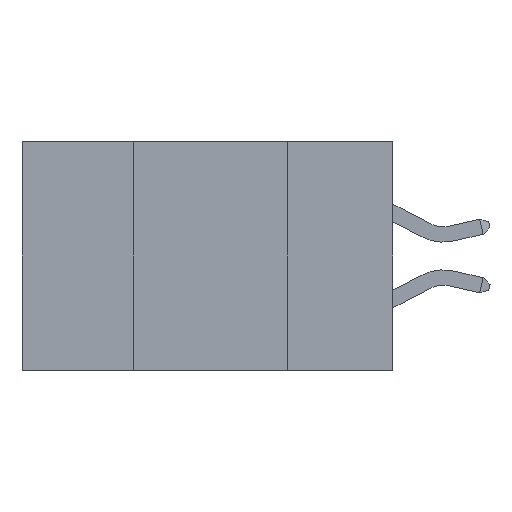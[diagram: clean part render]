
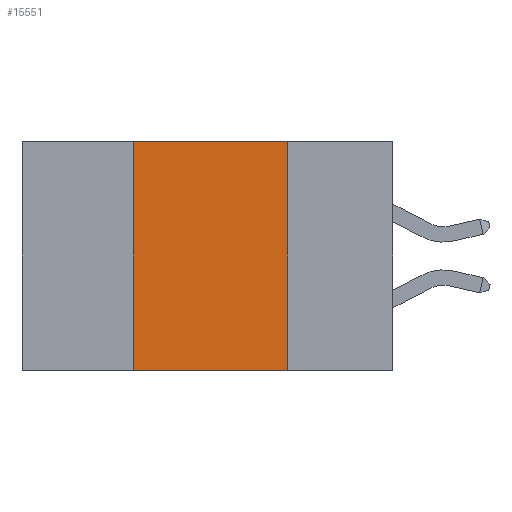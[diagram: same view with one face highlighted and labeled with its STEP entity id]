
A CAD part, left-side view. The second image highlights one B-rep face of the part: STEP entity #15551.
In plain terms, the highlighted planar face has unit normal (-1, 0, 0).
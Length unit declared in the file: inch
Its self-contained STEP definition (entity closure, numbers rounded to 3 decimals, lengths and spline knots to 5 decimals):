
#115 = CARTESIAN_POINT ( 'NONE',  ( 0., 0.17, 0. ) ) ;
#1339 = CARTESIAN_POINT ( 'NONE',  ( 0., 0.42, 0. ) ) ;
#2048 = LINE ( 'NONE', #1339, #14881 ) ;
#2567 = LINE ( 'NONE', #10502, #19224 ) ;
#3189 = EDGE_CURVE ( 'NONE', #14061, #12010, #2048, .T. ) ;
#3264 = VERTEX_POINT ( 'NONE', #9526 ) ;
#3727 = EDGE_LOOP ( 'NONE', ( #8977, #5033, #9612, #20613 ) ) ;
#4608 = LINE ( 'NONE', #18287, #12663 ) ;
#4973 = EDGE_CURVE ( 'NONE', #12010, #12367, #2567, .T. ) ;
#5033 = ORIENTED_EDGE ( 'NONE', *, *, #4973, .F. ) ;
#5217 = FACE_OUTER_BOUND ( 'NONE', #3727, .T. ) ;
#5993 = LINE ( 'NONE', #115, #10275 ) ;
#7487 = CARTESIAN_POINT ( 'NONE',  ( 0., 0.42, -0.37 ) ) ;
#8097 = DIRECTION ( 'NONE',  ( 0., 0., -1. ) ) ;
#8143 = CARTESIAN_POINT ( 'NONE',  ( 0., 0.6, 0. ) ) ;
#8977 = ORIENTED_EDGE ( 'NONE', *, *, #18829, .F. ) ;
#9085 = EDGE_CURVE ( 'NONE', #14061, #3264, #4608, .T. ) ;
#9526 = CARTESIAN_POINT ( 'NONE',  ( 0., 0.17, -0.37 ) ) ;
#9612 = ORIENTED_EDGE ( 'NONE', *, *, #3189, .F. ) ;
#9785 = DIRECTION ( 'NONE',  ( 0., 0., -1. ) ) ;
#10275 = VECTOR ( 'NONE', #8097, 39.37008 ) ;
#10502 = CARTESIAN_POINT ( 'NONE',  ( 0., 0.6, 0. ) ) ;
#10700 = CARTESIAN_POINT ( 'NONE',  ( 0., 0.17, 0. ) ) ;
#11210 = CARTESIAN_POINT ( 'NONE',  ( 0., 0.42, 0. ) ) ;
#12010 = VERTEX_POINT ( 'NONE', #11210 ) ;
#12367 = VERTEX_POINT ( 'NONE', #10700 ) ;
#12574 = DIRECTION ( 'NONE',  ( 0., 0., 1. ) ) ;
#12663 = VECTOR ( 'NONE', #16669, 39.37008 ) ;
#13837 = AXIS2_PLACEMENT_3D ( 'NONE', #8143, #19475, #9785 ) ;
#14061 = VERTEX_POINT ( 'NONE', #7487 ) ;
#14881 = VECTOR ( 'NONE', #12574, 39.37008 ) ;
#15371 = DIRECTION ( 'NONE',  ( 0., -1., 0. ) ) ;
#15551 = ADVANCED_FACE ( 'NONE', ( #5217 ), #19396, .F. ) ;
#16669 = DIRECTION ( 'NONE',  ( 0., -1., 0. ) ) ;
#18287 = CARTESIAN_POINT ( 'NONE',  ( 0., 0.6, -0.37 ) ) ;
#18829 = EDGE_CURVE ( 'NONE', #12367, #3264, #5993, .T. ) ;
#19224 = VECTOR ( 'NONE', #15371, 39.37008 ) ;
#19396 = PLANE ( 'NONE',  #13837 ) ;
#19475 = DIRECTION ( 'NONE',  ( 1., 0., 0. ) ) ;
#20613 = ORIENTED_EDGE ( 'NONE', *, *, #9085, .T. ) ;
